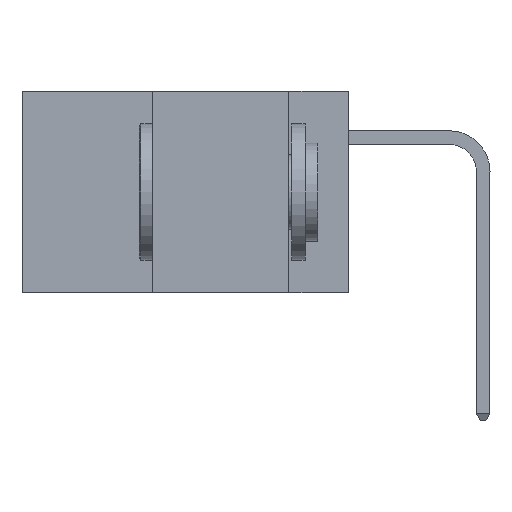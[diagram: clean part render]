
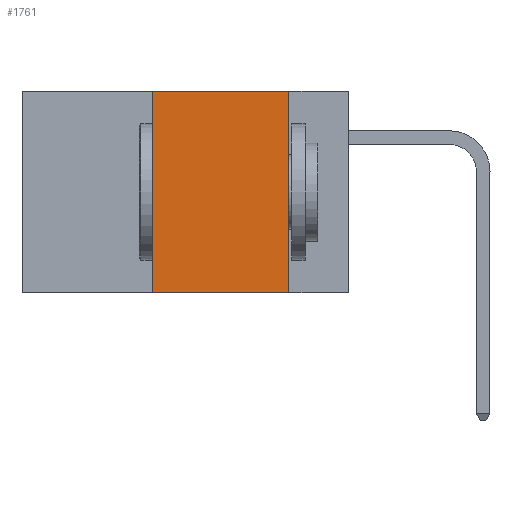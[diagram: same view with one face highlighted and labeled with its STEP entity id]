
A CAD part, left-side view. The second image highlights one B-rep face of the part: STEP entity #1761.
In plain terms, the highlighted planar face has unit normal (-1, 0, 0).
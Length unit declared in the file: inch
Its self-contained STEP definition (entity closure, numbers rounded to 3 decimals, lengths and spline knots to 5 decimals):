
#101 = CARTESIAN_POINT ( 'NONE',  ( 0., 0.36, 0. ) ) ;
#399 = VECTOR ( 'NONE', #7342, 39.37008 ) ;
#421 = ORIENTED_EDGE ( 'NONE', *, *, #15783, .T. ) ;
#536 = EDGE_CURVE ( 'NONE', #2970, #2827, #11124, .T. ) ;
#1365 = LINE ( 'NONE', #3242, #5589 ) ;
#1521 = VECTOR ( 'NONE', #14102, 39.37008 ) ;
#1761 = ADVANCED_FACE ( 'NONE', ( #9159 ), #12740, .F. ) ;
#1776 = DIRECTION ( 'NONE',  ( 0., 0., -1. ) ) ;
#2443 = ORIENTED_EDGE ( 'NONE', *, *, #536, .F. ) ;
#2696 = VECTOR ( 'NONE', #5432, 39.37008 ) ;
#2827 = VERTEX_POINT ( 'NONE', #7895 ) ;
#2970 = VERTEX_POINT ( 'NONE', #15432 ) ;
#3079 = CARTESIAN_POINT ( 'NONE',  ( 0., 0.6, 0. ) ) ;
#3242 = CARTESIAN_POINT ( 'NONE',  ( 0., 0.11, 0. ) ) ;
#3702 = VERTEX_POINT ( 'NONE', #12728 ) ;
#4114 = ORIENTED_EDGE ( 'NONE', *, *, #5517, .F. ) ;
#4322 = CARTESIAN_POINT ( 'NONE',  ( 0., 0.6, 0. ) ) ;
#4561 = DIRECTION ( 'NONE',  ( 0., 0., -1. ) ) ;
#5432 = DIRECTION ( 'NONE',  ( 0., -1., 0. ) ) ;
#5517 = EDGE_CURVE ( 'NONE', #3702, #2970, #12273, .T. ) ;
#5589 = VECTOR ( 'NONE', #4561, 39.37008 ) ;
#7162 = CARTESIAN_POINT ( 'NONE',  ( 0., 0.11, -0.37 ) ) ;
#7342 = DIRECTION ( 'NONE',  ( 0., 0., 1. ) ) ;
#7895 = CARTESIAN_POINT ( 'NONE',  ( 0., 0.11, 0. ) ) ;
#9159 = FACE_OUTER_BOUND ( 'NONE', #9168, .T. ) ;
#9168 = EDGE_LOOP ( 'NONE', ( #12652, #2443, #4114, #421 ) ) ;
#11124 = LINE ( 'NONE', #4322, #1521 ) ;
#12273 = LINE ( 'NONE', #101, #399 ) ;
#12501 = AXIS2_PLACEMENT_3D ( 'NONE', #3079, #13963, #1776 ) ;
#12652 = ORIENTED_EDGE ( 'NONE', *, *, #14121, .F. ) ;
#12728 = CARTESIAN_POINT ( 'NONE',  ( 0., 0.36, -0.37 ) ) ;
#12740 = PLANE ( 'NONE',  #12501 ) ;
#12766 = CARTESIAN_POINT ( 'NONE',  ( 0., 0.6, -0.37 ) ) ;
#13322 = VERTEX_POINT ( 'NONE', #7162 ) ;
#13962 = LINE ( 'NONE', #12766, #2696 ) ;
#13963 = DIRECTION ( 'NONE',  ( 1., 0., 0. ) ) ;
#14102 = DIRECTION ( 'NONE',  ( 0., -1., 0. ) ) ;
#14121 = EDGE_CURVE ( 'NONE', #2827, #13322, #1365, .T. ) ;
#15432 = CARTESIAN_POINT ( 'NONE',  ( 0., 0.36, 0. ) ) ;
#15783 = EDGE_CURVE ( 'NONE', #3702, #13322, #13962, .T. ) ;
